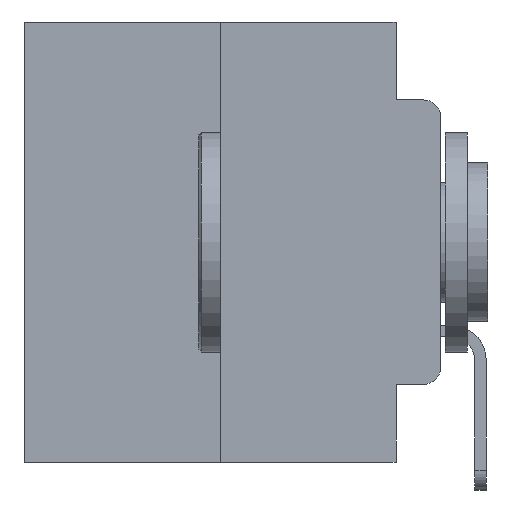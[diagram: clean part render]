
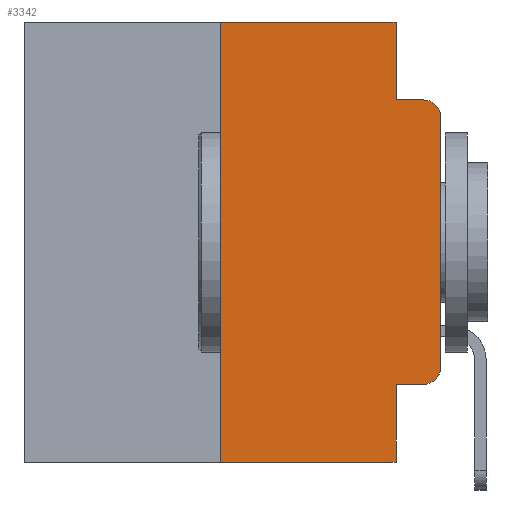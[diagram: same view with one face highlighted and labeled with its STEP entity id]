
A CAD part, left-side view. The second image highlights one B-rep face of the part: STEP entity #3342.
In plain terms, the highlighted planar face has unit normal (-1, 0, 0).
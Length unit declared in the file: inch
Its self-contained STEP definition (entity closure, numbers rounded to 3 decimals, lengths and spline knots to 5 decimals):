
#196 = PLANE ( 'NONE',  #14783 ) ;
#521 = VERTEX_POINT ( 'NONE', #2308 ) ;
#615 = ORIENTED_EDGE ( 'NONE', *, *, #7327, .T. ) ;
#718 = LINE ( 'NONE', #18221, #1394 ) ;
#833 = DIRECTION ( 'NONE',  ( 0., -1., 0. ) ) ;
#1067 = CARTESIAN_POINT ( 'NONE',  ( 0., 0.02, -0.4115 ) ) ;
#1394 = VECTOR ( 'NONE', #3384, 39.37008 ) ;
#1703 = LINE ( 'NONE', #14804, #24777 ) ;
#2088 = DIRECTION ( 'NONE',  ( 0., 0., -1. ) ) ;
#2308 = CARTESIAN_POINT ( 'NONE',  ( 0., 0.25, 0. ) ) ;
#2834 = CARTESIAN_POINT ( 'NONE',  ( 0., 0.051, -0.4115 ) ) ;
#2954 = DIRECTION ( 'NONE',  ( -1., 0., 0. ) ) ;
#3121 = ORIENTED_EDGE ( 'NONE', *, *, #27178, .T. ) ;
#3342 = ADVANCED_FACE ( 'NONE', ( #19042 ), #196, .F. ) ;
#3384 = DIRECTION ( 'NONE',  ( 0., -1., 0. ) ) ;
#3832 = DIRECTION ( 'NONE',  ( 0., 0., -1. ) ) ;
#3846 = DIRECTION ( 'NONE',  ( 0., -1., 0. ) ) ;
#3880 = VERTEX_POINT ( 'NONE', #10915 ) ;
#4019 = DIRECTION ( 'NONE',  ( 0., 0., 1. ) ) ;
#4132 = CARTESIAN_POINT ( 'NONE',  ( 0., 0.051, 0. ) ) ;
#4184 = DIRECTION ( 'NONE',  ( 0., 0., -1. ) ) ;
#4274 = CIRCLE ( 'NONE', #17420, 0.02 ) ;
#4399 = ORIENTED_EDGE ( 'NONE', *, *, #4688, .T. ) ;
#4688 = EDGE_CURVE ( 'NONE', #17353, #13712, #11905, .T. ) ;
#4821 = EDGE_CURVE ( 'NONE', #19795, #11545, #8270, .T. ) ;
#4999 = EDGE_CURVE ( 'NONE', #24709, #19795, #13264, .T. ) ;
#5020 = DIRECTION ( 'NONE',  ( 0., 0., 1. ) ) ;
#5266 = DIRECTION ( 'NONE',  ( 0., 0., -1. ) ) ;
#5839 = LINE ( 'NONE', #14816, #25890 ) ;
#5972 = LINE ( 'NONE', #18694, #22035 ) ;
#6243 = ORIENTED_EDGE ( 'NONE', *, *, #20818, .T. ) ;
#6654 = CARTESIAN_POINT ( 'NONE',  ( 0., 0.02, -0.0885 ) ) ;
#6810 = VERTEX_POINT ( 'NONE', #13191 ) ;
#7229 = CARTESIAN_POINT ( 'NONE',  ( 0., 0.02, -0.3915 ) ) ;
#7327 = EDGE_CURVE ( 'NONE', #13712, #3880, #24233, .T. ) ;
#8270 = LINE ( 'NONE', #24206, #24689 ) ;
#8726 = ORIENTED_EDGE ( 'NONE', *, *, #19687, .F. ) ;
#8749 = CARTESIAN_POINT ( 'NONE',  ( 0., 0.473, 0. ) ) ;
#8757 = DIRECTION ( 'NONE',  ( -1., 0., 0. ) ) ;
#10284 = ORIENTED_EDGE ( 'NONE', *, *, #22651, .T. ) ;
#10743 = ORIENTED_EDGE ( 'NONE', *, *, #4999, .F. ) ;
#10900 = DIRECTION ( 'NONE',  ( 1., 0., 0. ) ) ;
#10915 = CARTESIAN_POINT ( 'NONE',  ( 0., 0., -0.1085 ) ) ;
#11536 = CARTESIAN_POINT ( 'NONE',  ( 0., 0.473, -0.5 ) ) ;
#11545 = VERTEX_POINT ( 'NONE', #6654 ) ;
#11905 = CIRCLE ( 'NONE', #22671, 0.02 ) ;
#12063 = VERTEX_POINT ( 'NONE', #25338 ) ;
#12077 = VECTOR ( 'NONE', #833, 39.37008 ) ;
#13191 = CARTESIAN_POINT ( 'NONE',  ( 0., 0.25, -0.5 ) ) ;
#13264 = LINE ( 'NONE', #19352, #16280 ) ;
#13687 = CARTESIAN_POINT ( 'NONE',  ( 0., 0., 0. ) ) ;
#13712 = VERTEX_POINT ( 'NONE', #18210 ) ;
#13977 = EDGE_CURVE ( 'NONE', #23837, #12063, #1703, .T. ) ;
#14783 = AXIS2_PLACEMENT_3D ( 'NONE', #8749, #10900, #4184 ) ;
#14804 = CARTESIAN_POINT ( 'NONE',  ( 0., 0.051, 0. ) ) ;
#14816 = CARTESIAN_POINT ( 'NONE',  ( 0., 0.25, 0. ) ) ;
#16280 = VECTOR ( 'NONE', #2088, 39.37008 ) ;
#17056 = CARTESIAN_POINT ( 'NONE',  ( 0., 0.051, -0.0885 ) ) ;
#17143 = DIRECTION ( 'NONE',  ( 0., 0., -1. ) ) ;
#17353 = VERTEX_POINT ( 'NONE', #1067 ) ;
#17420 = AXIS2_PLACEMENT_3D ( 'NONE', #25699, #8757, #17143 ) ;
#18194 = ORIENTED_EDGE ( 'NONE', *, *, #26967, .F. ) ;
#18210 = CARTESIAN_POINT ( 'NONE',  ( 0., 0., -0.3915 ) ) ;
#18221 = CARTESIAN_POINT ( 'NONE',  ( 0., 0.051, -0.4115 ) ) ;
#18694 = CARTESIAN_POINT ( 'NONE',  ( 0., 0.473, 0. ) ) ;
#19042 = FACE_OUTER_BOUND ( 'NONE', #21442, .T. ) ;
#19352 = CARTESIAN_POINT ( 'NONE',  ( 0., 0.051, 0. ) ) ;
#19654 = ORIENTED_EDGE ( 'NONE', *, *, #13977, .F. ) ;
#19687 = EDGE_CURVE ( 'NONE', #6810, #521, #5839, .T. ) ;
#19795 = VERTEX_POINT ( 'NONE', #17056 ) ;
#20175 = VECTOR ( 'NONE', #5020, 39.37008 ) ;
#20818 = EDGE_CURVE ( 'NONE', #23837, #17353, #718, .T. ) ;
#21442 = EDGE_LOOP ( 'NONE', ( #615, #3121, #22249, #10743, #18194, #8726, #10284, #19654, #6243, #4399 ) ) ;
#22035 = VECTOR ( 'NONE', #3846, 39.37008 ) ;
#22249 = ORIENTED_EDGE ( 'NONE', *, *, #4821, .F. ) ;
#22651 = EDGE_CURVE ( 'NONE', #6810, #12063, #24184, .T. ) ;
#22671 = AXIS2_PLACEMENT_3D ( 'NONE', #7229, #2954, #5266 ) ;
#23837 = VERTEX_POINT ( 'NONE', #2834 ) ;
#24184 = LINE ( 'NONE', #11536, #12077 ) ;
#24206 = CARTESIAN_POINT ( 'NONE',  ( 0., 0.051, -0.0885 ) ) ;
#24233 = LINE ( 'NONE', #13687, #20175 ) ;
#24689 = VECTOR ( 'NONE', #25569, 39.37008 ) ;
#24709 = VERTEX_POINT ( 'NONE', #4132 ) ;
#24777 = VECTOR ( 'NONE', #3832, 39.37008 ) ;
#25338 = CARTESIAN_POINT ( 'NONE',  ( 0., 0.051, -0.5 ) ) ;
#25569 = DIRECTION ( 'NONE',  ( 0., -1., 0. ) ) ;
#25699 = CARTESIAN_POINT ( 'NONE',  ( 0., 0.02, -0.1085 ) ) ;
#25890 = VECTOR ( 'NONE', #4019, 39.37008 ) ;
#26967 = EDGE_CURVE ( 'NONE', #521, #24709, #5972, .T. ) ;
#27178 = EDGE_CURVE ( 'NONE', #3880, #11545, #4274, .T. ) ;
